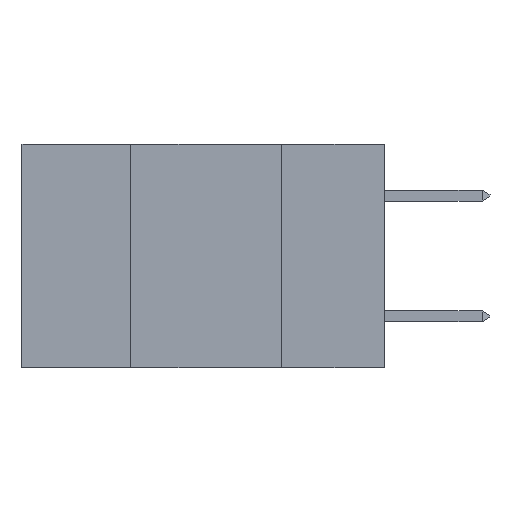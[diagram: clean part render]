
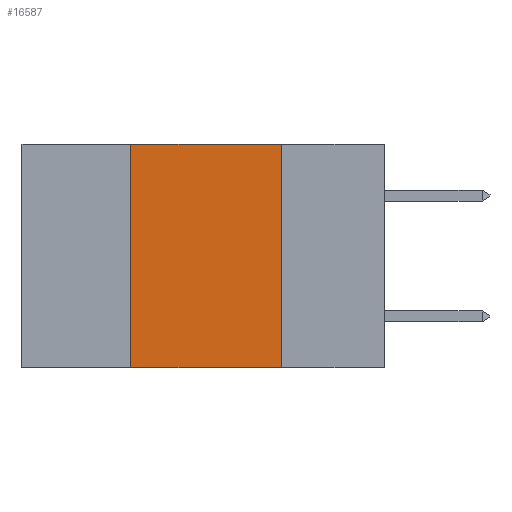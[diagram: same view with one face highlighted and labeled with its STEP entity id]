
A CAD part, left-side view. The second image highlights one B-rep face of the part: STEP entity #16587.
In plain terms, the highlighted planar face has unit normal (-1, 0, 0).
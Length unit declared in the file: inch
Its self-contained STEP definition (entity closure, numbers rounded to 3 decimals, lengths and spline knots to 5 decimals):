
#1989 = EDGE_CURVE ( 'NONE', #14688, #12163, #16848, .T. ) ;
#2599 = ORIENTED_EDGE ( 'NONE', *, *, #18599, .F. ) ;
#2967 = EDGE_LOOP ( 'NONE', ( #6031, #2599, #10845, #5553 ) ) ;
#3729 = VECTOR ( 'NONE', #9336, 39.37008 ) ;
#3749 = FACE_OUTER_BOUND ( 'NONE', #2967, .T. ) ;
#5553 = ORIENTED_EDGE ( 'NONE', *, *, #1989, .T. ) ;
#5563 = CARTESIAN_POINT ( 'NONE',  ( 0., 0.42, 0. ) ) ;
#5755 = LINE ( 'NONE', #5563, #3729 ) ;
#5758 = EDGE_CURVE ( 'NONE', #20763, #12163, #7633, .T. ) ;
#6031 = ORIENTED_EDGE ( 'NONE', *, *, #5758, .F. ) ;
#7126 = CARTESIAN_POINT ( 'NONE',  ( 0., 0.42, 0. ) ) ;
#7385 = DIRECTION ( 'NONE',  ( 0., 0., -1. ) ) ;
#7389 = LINE ( 'NONE', #9980, #20145 ) ;
#7633 = LINE ( 'NONE', #11783, #15767 ) ;
#8753 = VECTOR ( 'NONE', #14029, 39.37008 ) ;
#9255 = CARTESIAN_POINT ( 'NONE',  ( 0., 0.6, 0. ) ) ;
#9336 = DIRECTION ( 'NONE',  ( 0., 0., 1. ) ) ;
#9980 = CARTESIAN_POINT ( 'NONE',  ( 0., 0.6, 0. ) ) ;
#10845 = ORIENTED_EDGE ( 'NONE', *, *, #16653, .F. ) ;
#11740 = DIRECTION ( 'NONE',  ( 0., -1., 0. ) ) ;
#11783 = CARTESIAN_POINT ( 'NONE',  ( 0., 0.17, 0. ) ) ;
#12163 = VERTEX_POINT ( 'NONE', #16891 ) ;
#12884 = CARTESIAN_POINT ( 'NONE',  ( 0., 0.42, -0.37 ) ) ;
#13118 = PLANE ( 'NONE',  #19862 ) ;
#13188 = DIRECTION ( 'NONE',  ( 1., 0., 0. ) ) ;
#14029 = DIRECTION ( 'NONE',  ( 0., -1., 0. ) ) ;
#14688 = VERTEX_POINT ( 'NONE', #12884 ) ;
#15767 = VECTOR ( 'NONE', #17389, 39.37008 ) ;
#15808 = CARTESIAN_POINT ( 'NONE',  ( 0., 0.6, -0.37 ) ) ;
#16587 = ADVANCED_FACE ( 'NONE', ( #3749 ), #13118, .F. ) ;
#16653 = EDGE_CURVE ( 'NONE', #14688, #20767, #5755, .T. ) ;
#16848 = LINE ( 'NONE', #15808, #8753 ) ;
#16891 = CARTESIAN_POINT ( 'NONE',  ( 0., 0.17, -0.37 ) ) ;
#17389 = DIRECTION ( 'NONE',  ( 0., 0., -1. ) ) ;
#18599 = EDGE_CURVE ( 'NONE', #20767, #20763, #7389, .T. ) ;
#19862 = AXIS2_PLACEMENT_3D ( 'NONE', #9255, #13188, #7385 ) ;
#20145 = VECTOR ( 'NONE', #11740, 39.37008 ) ;
#20763 = VERTEX_POINT ( 'NONE', #21483 ) ;
#20767 = VERTEX_POINT ( 'NONE', #7126 ) ;
#21483 = CARTESIAN_POINT ( 'NONE',  ( 0., 0.17, 0. ) ) ;
